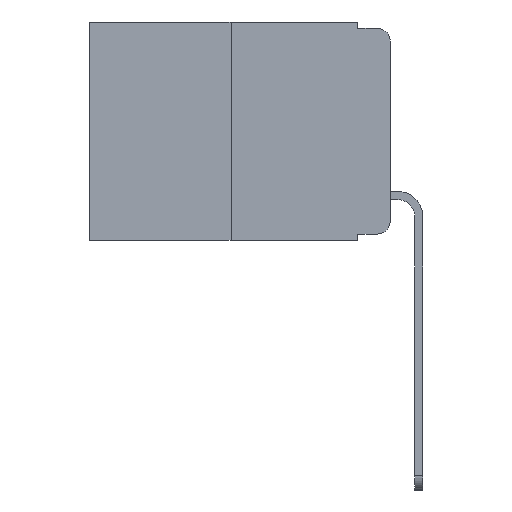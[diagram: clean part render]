
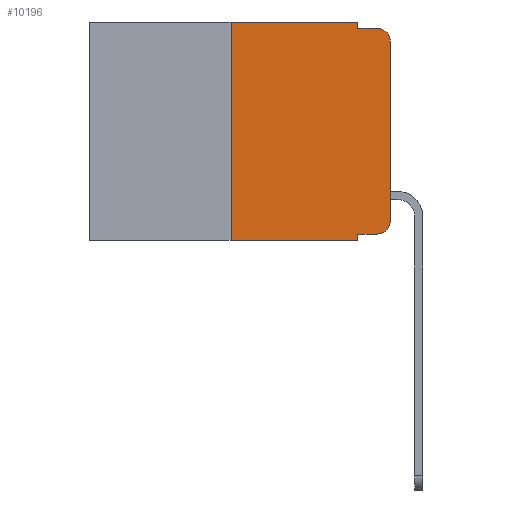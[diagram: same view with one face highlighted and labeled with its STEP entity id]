
A CAD part, left-side view. The second image highlights one B-rep face of the part: STEP entity #10196.
In plain terms, the highlighted planar face has unit normal (-1, 0, 0).
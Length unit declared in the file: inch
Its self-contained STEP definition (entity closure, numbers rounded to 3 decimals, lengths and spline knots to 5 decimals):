
#24 = CARTESIAN_POINT ( 'NONE',  ( 0., 0.473, 0. ) ) ;
#63 = DIRECTION ( 'NONE',  ( 0., -1., 0. ) ) ;
#82 = ORIENTED_EDGE ( 'NONE', *, *, #2118, .F. ) ;
#399 = AXIS2_PLACEMENT_3D ( 'NONE', #24, #8259, #2004 ) ;
#444 = DIRECTION ( 'NONE',  ( 0., 0., -1. ) ) ;
#526 = LINE ( 'NONE', #558, #6711 ) ;
#558 = CARTESIAN_POINT ( 'NONE',  ( 0., 0.051, -0.333 ) ) ;
#606 = DIRECTION ( 'NONE',  ( 0., 0., 1. ) ) ;
#1048 = PLANE ( 'NONE',  #399 ) ;
#1072 = EDGE_CURVE ( 'NONE', #3708, #6562, #3877, .T. ) ;
#1155 = CARTESIAN_POINT ( 'NONE',  ( 0., 0.051, -0.333 ) ) ;
#1187 = DIRECTION ( 'NONE',  ( 0., 0., -1. ) ) ;
#1278 = DIRECTION ( 'NONE',  ( -1., 0., 0. ) ) ;
#1285 = EDGE_CURVE ( 'NONE', #6014, #4059, #10171, .T. ) ;
#1289 = CARTESIAN_POINT ( 'NONE',  ( 0., 0.02, -0.03 ) ) ;
#1325 = CARTESIAN_POINT ( 'NONE',  ( 0., 0.051, 0. ) ) ;
#1374 = CARTESIAN_POINT ( 'NONE',  ( 0., 0.051, 0. ) ) ;
#1464 = LINE ( 'NONE', #2607, #3593 ) ;
#1658 = DIRECTION ( 'NONE',  ( 0., -1., 0. ) ) ;
#2004 = DIRECTION ( 'NONE',  ( 0., 0., -1. ) ) ;
#2082 = EDGE_CURVE ( 'NONE', #9782, #5451, #4617, .T. ) ;
#2103 = EDGE_CURVE ( 'NONE', #5451, #5194, #4358, .T. ) ;
#2118 = EDGE_CURVE ( 'NONE', #8220, #5194, #5933, .T. ) ;
#2121 = EDGE_CURVE ( 'NONE', #4059, #8220, #1464, .T. ) ;
#2154 = EDGE_CURVE ( 'NONE', #3708, #6014, #5258, .T. ) ;
#2170 = EDGE_CURVE ( 'NONE', #8296, #6562, #6929, .T. ) ;
#2172 = EDGE_CURVE ( 'NONE', #8296, #8139, #526, .T. ) ;
#2194 = EDGE_CURVE ( 'NONE', #8139, #9782, #6234, .T. ) ;
#2369 = VECTOR ( 'NONE', #5716, 39.37008 ) ;
#2382 = CARTESIAN_POINT ( 'NONE',  ( 0., 0.051, -0.01 ) ) ;
#2384 = ORIENTED_EDGE ( 'NONE', *, *, #2103, .T. ) ;
#2569 = DIRECTION ( 'NONE',  ( -1., 0., 0. ) ) ;
#2606 = DIRECTION ( 'NONE',  ( 0., 0., -1. ) ) ;
#2607 = CARTESIAN_POINT ( 'NONE',  ( 0., 0.051, 0. ) ) ;
#2830 = CARTESIAN_POINT ( 'NONE',  ( 0., 0.25, 0. ) ) ;
#2994 = DIRECTION ( 'NONE',  ( 0., -1., 0. ) ) ;
#3035 = CARTESIAN_POINT ( 'NONE',  ( 0., 0.02, -0.313 ) ) ;
#3265 = DIRECTION ( 'NONE',  ( 0., 0., -1. ) ) ;
#3492 = ORIENTED_EDGE ( 'NONE', *, *, #1072, .T. ) ;
#3593 = VECTOR ( 'NONE', #2606, 39.37008 ) ;
#3708 = VERTEX_POINT ( 'NONE', #5309 ) ;
#3831 = VECTOR ( 'NONE', #1658, 39.37008 ) ;
#3877 = LINE ( 'NONE', #7737, #5743 ) ;
#4059 = VERTEX_POINT ( 'NONE', #1374 ) ;
#4098 = CARTESIAN_POINT ( 'NONE',  ( 0., 0., -0.313 ) ) ;
#4247 = VECTOR ( 'NONE', #63, 39.37008 ) ;
#4312 = EDGE_LOOP ( 'NONE', ( #4376, #2384, #82, #6838, #9003, #5394, #3492, #7992, #8218, #4768 ) ) ;
#4318 = CARTESIAN_POINT ( 'NONE',  ( 0., 0., 0. ) ) ;
#4358 = CIRCLE ( 'NONE', #7554, 0.02 ) ;
#4376 = ORIENTED_EDGE ( 'NONE', *, *, #2082, .T. ) ;
#4497 = FACE_OUTER_BOUND ( 'NONE', #4312, .T. ) ;
#4617 = LINE ( 'NONE', #4318, #2369 ) ;
#4768 = ORIENTED_EDGE ( 'NONE', *, *, #2194, .T. ) ;
#5014 = VECTOR ( 'NONE', #1187, 39.37008 ) ;
#5194 = VERTEX_POINT ( 'NONE', #5989 ) ;
#5258 = LINE ( 'NONE', #2830, #8867 ) ;
#5309 = CARTESIAN_POINT ( 'NONE',  ( 0., 0.25, -0.343 ) ) ;
#5394 = ORIENTED_EDGE ( 'NONE', *, *, #2154, .F. ) ;
#5451 = VERTEX_POINT ( 'NONE', #5668 ) ;
#5668 = CARTESIAN_POINT ( 'NONE',  ( 0., 0., -0.03 ) ) ;
#5716 = DIRECTION ( 'NONE',  ( 0., 0., 1. ) ) ;
#5743 = VECTOR ( 'NONE', #5958, 39.37008 ) ;
#5933 = LINE ( 'NONE', #2382, #3831 ) ;
#5958 = DIRECTION ( 'NONE',  ( 0., -1., 0. ) ) ;
#5989 = CARTESIAN_POINT ( 'NONE',  ( 0., 0.02, -0.01 ) ) ;
#6014 = VERTEX_POINT ( 'NONE', #6625 ) ;
#6234 = CIRCLE ( 'NONE', #8644, 0.02 ) ;
#6562 = VERTEX_POINT ( 'NONE', #8391 ) ;
#6625 = CARTESIAN_POINT ( 'NONE',  ( 0., 0.25, 0. ) ) ;
#6711 = VECTOR ( 'NONE', #2994, 39.37008 ) ;
#6838 = ORIENTED_EDGE ( 'NONE', *, *, #2121, .F. ) ;
#6929 = LINE ( 'NONE', #1325, #5014 ) ;
#7554 = AXIS2_PLACEMENT_3D ( 'NONE', #1289, #1278, #444 ) ;
#7737 = CARTESIAN_POINT ( 'NONE',  ( 0., 0.473, -0.343 ) ) ;
#7992 = ORIENTED_EDGE ( 'NONE', *, *, #2170, .F. ) ;
#8139 = VERTEX_POINT ( 'NONE', #8919 ) ;
#8218 = ORIENTED_EDGE ( 'NONE', *, *, #2172, .T. ) ;
#8220 = VERTEX_POINT ( 'NONE', #9009 ) ;
#8259 = DIRECTION ( 'NONE',  ( 1., 0., 0. ) ) ;
#8296 = VERTEX_POINT ( 'NONE', #1155 ) ;
#8391 = CARTESIAN_POINT ( 'NONE',  ( 0., 0.051, -0.343 ) ) ;
#8470 = CARTESIAN_POINT ( 'NONE',  ( 0., 0.473, 0. ) ) ;
#8644 = AXIS2_PLACEMENT_3D ( 'NONE', #3035, #2569, #3265 ) ;
#8867 = VECTOR ( 'NONE', #606, 39.37008 ) ;
#8919 = CARTESIAN_POINT ( 'NONE',  ( 0., 0.02, -0.333 ) ) ;
#9003 = ORIENTED_EDGE ( 'NONE', *, *, #1285, .F. ) ;
#9009 = CARTESIAN_POINT ( 'NONE',  ( 0., 0.051, -0.01 ) ) ;
#9782 = VERTEX_POINT ( 'NONE', #4098 ) ;
#10171 = LINE ( 'NONE', #8470, #4247 ) ;
#10196 = ADVANCED_FACE ( 'NONE', ( #4497 ), #1048, .F. ) ;
